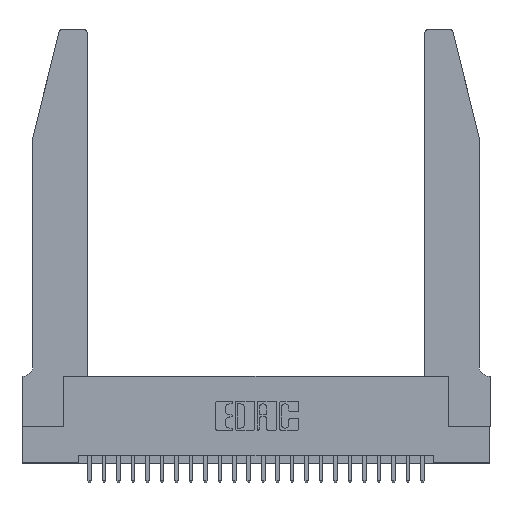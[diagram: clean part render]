
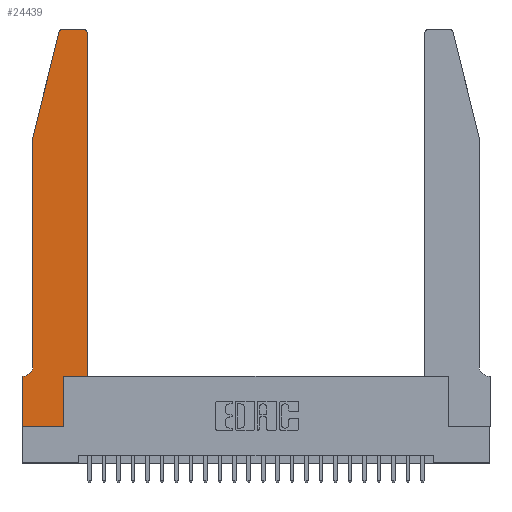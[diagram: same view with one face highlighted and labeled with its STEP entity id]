
A CAD part, top view. The second image highlights one B-rep face of the part: STEP entity #24439.
In plain terms, the highlighted planar face has unit normal (0, 0, 1).
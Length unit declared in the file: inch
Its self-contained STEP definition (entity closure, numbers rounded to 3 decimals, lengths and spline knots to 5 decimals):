
#149 = CARTESIAN_POINT ( 'NONE',  ( 0.4205, 2.75, 0.37 ) ) ;
#637 = VERTEX_POINT ( 'NONE', #7300 ) ;
#642 = AXIS2_PLACEMENT_3D ( 'NONE', #14940, #10970, #20933 ) ;
#1613 = VECTOR ( 'NONE', #25043, 39.37008 ) ;
#1618 = DIRECTION ( 'NONE',  ( 1., 0., 0. ) ) ;
#1710 = VECTOR ( 'NONE', #6680, 39.37008 ) ;
#2078 = EDGE_CURVE ( 'NONE', #21010, #8955, #11226, .T. ) ;
#2170 = CARTESIAN_POINT ( 'NONE',  ( 0., 0.35, 0.37 ) ) ;
#2839 = LINE ( 'NONE', #24958, #12929 ) ;
#3309 = DIRECTION ( 'NONE',  ( 0., 0., -1. ) ) ;
#3451 = VERTEX_POINT ( 'NONE', #17751 ) ;
#3576 = DIRECTION ( 'NONE',  ( -1., 0., 0. ) ) ;
#4223 = EDGE_CURVE ( 'NONE', #8955, #25640, #12965, .T. ) ;
#4373 = CARTESIAN_POINT ( 'NONE',  ( 0.2865, 0.35, 0.37 ) ) ;
#4541 = VECTOR ( 'NONE', #18914, 39.37008 ) ;
#4555 = AXIS2_PLACEMENT_3D ( 'NONE', #10861, #18971, #19320 ) ;
#5529 = CARTESIAN_POINT ( 'NONE',  ( 0.0755, 2., 0.37 ) ) ;
#5613 = EDGE_CURVE ( 'NONE', #10034, #25306, #20818, .T. ) ;
#5662 = CARTESIAN_POINT ( 'NONE',  ( 0.284, 2.75, 0.37 ) ) ;
#6236 = LINE ( 'NONE', #5529, #16347 ) ;
#6680 = DIRECTION ( 'NONE',  ( 0., 1., 0. ) ) ;
#6697 = VECTOR ( 'NONE', #3576, 39.37008 ) ;
#6844 = EDGE_CURVE ( 'NONE', #18125, #24211, #19316, .T. ) ;
#7100 = CARTESIAN_POINT ( 'NONE',  ( 0.2865, 0., 0.37 ) ) ;
#7226 = AXIS2_PLACEMENT_3D ( 'NONE', #2170, #18486, #14240 ) ;
#7234 = CARTESIAN_POINT ( 'NONE',  ( 0.0055, 0.42, 0.37 ) ) ;
#7300 = CARTESIAN_POINT ( 'NONE',  ( 0.0755, 2., 0.37 ) ) ;
#7358 = PLANE ( 'NONE',  #7226 ) ;
#7670 = ORIENTED_EDGE ( 'NONE', *, *, #10419, .T. ) ;
#7861 = AXIS2_PLACEMENT_3D ( 'NONE', #7234, #3309, #21483 ) ;
#7967 = LINE ( 'NONE', #15758, #6697 ) ;
#8093 = CARTESIAN_POINT ( 'NONE',  ( 0.0755, 0.35, 0.37 ) ) ;
#8360 = EDGE_CURVE ( 'NONE', #25306, #24213, #19548, .T. ) ;
#8680 = CARTESIAN_POINT ( 'NONE',  ( 0.25487, 2.72718, 0.37 ) ) ;
#8682 = ORIENTED_EDGE ( 'NONE', *, *, #2078, .T. ) ;
#8781 = ORIENTED_EDGE ( 'NONE', *, *, #20488, .T. ) ;
#8790 = ORIENTED_EDGE ( 'NONE', *, *, #19076, .T. ) ;
#8955 = VERTEX_POINT ( 'NONE', #16636 ) ;
#9292 = DIRECTION ( 'NONE',  ( 0., 1., 0. ) ) ;
#9666 = CIRCLE ( 'NONE', #4555, 0.03 ) ;
#9838 = FACE_OUTER_BOUND ( 'NONE', #14586, .T. ) ;
#10034 = VERTEX_POINT ( 'NONE', #7100 ) ;
#10419 = EDGE_CURVE ( 'NONE', #22791, #20185, #9666, .T. ) ;
#10783 = DIRECTION ( 'NONE',  ( 1., 0., 0. ) ) ;
#10861 = CARTESIAN_POINT ( 'NONE',  ( 0.4205, 2.72, 0.37 ) ) ;
#10890 = ORIENTED_EDGE ( 'NONE', *, *, #8360, .T. ) ;
#10970 = DIRECTION ( 'NONE',  ( 0., 0., 1. ) ) ;
#11226 = LINE ( 'NONE', #8093, #4541 ) ;
#11276 = DIRECTION ( 'NONE',  ( 0., -1., 0. ) ) ;
#11474 = EDGE_CURVE ( 'NONE', #3451, #21010, #26013, .T. ) ;
#12108 = EDGE_CURVE ( 'NONE', #24213, #22791, #19376, .T. ) ;
#12929 = VECTOR ( 'NONE', #11276, 39.37008 ) ;
#12965 = LINE ( 'NONE', #19267, #1613 ) ;
#13298 = DIRECTION ( 'NONE',  ( -0.239, -0.971, 0. ) ) ;
#13448 = ORIENTED_EDGE ( 'NONE', *, *, #4223, .T. ) ;
#13584 = ORIENTED_EDGE ( 'NONE', *, *, #5613, .T. ) ;
#14240 = DIRECTION ( 'NONE',  ( 1., 0., 0. ) ) ;
#14586 = EDGE_LOOP ( 'NONE', ( #8790, #24804, #21444, #8781, #20451, #8682, #13448, #21545, #13584, #10890, #24182, #7670 ) ) ;
#14940 = CARTESIAN_POINT ( 'NONE',  ( 0.284, 2.72, 0.37 ) ) ;
#15050 = CARTESIAN_POINT ( 'NONE',  ( 0.4505, 0.35, 0.37 ) ) ;
#15729 = CARTESIAN_POINT ( 'NONE',  ( 0., 0., 0.37 ) ) ;
#15758 = CARTESIAN_POINT ( 'NONE',  ( 0.2605, 2.75, 0.37 ) ) ;
#16347 = VECTOR ( 'NONE', #13298, 39.37008 ) ;
#16636 = CARTESIAN_POINT ( 'NONE',  ( 0., 0.35, 0.37 ) ) ;
#17296 = CARTESIAN_POINT ( 'NONE',  ( 0., 0., 0.37 ) ) ;
#17751 = CARTESIAN_POINT ( 'NONE',  ( 0.0755, 0.42, 0.37 ) ) ;
#18125 = VERTEX_POINT ( 'NONE', #5662 ) ;
#18486 = DIRECTION ( 'NONE',  ( 0., 0., 1. ) ) ;
#18597 = VECTOR ( 'NONE', #10783, 39.37008 ) ;
#18914 = DIRECTION ( 'NONE',  ( -1., 0., 0. ) ) ;
#18971 = DIRECTION ( 'NONE',  ( 0., 0., 1. ) ) ;
#19076 = EDGE_CURVE ( 'NONE', #20185, #18125, #7967, .T. ) ;
#19267 = CARTESIAN_POINT ( 'NONE',  ( 0., 0., 0.37 ) ) ;
#19316 = CIRCLE ( 'NONE', #642, 0.03 ) ;
#19320 = DIRECTION ( 'NONE',  ( 1., 0., 0. ) ) ;
#19331 = CARTESIAN_POINT ( 'NONE',  ( 0.2865, 0.35, 0.37 ) ) ;
#19376 = LINE ( 'NONE', #15050, #1710 ) ;
#19548 = LINE ( 'NONE', #22826, #18597 ) ;
#19781 = EDGE_CURVE ( 'NONE', #25640, #10034, #21165, .T. ) ;
#20185 = VERTEX_POINT ( 'NONE', #149 ) ;
#20211 = CARTESIAN_POINT ( 'NONE',  ( 0.0055, 0.35, 0.37 ) ) ;
#20451 = ORIENTED_EDGE ( 'NONE', *, *, #11474, .T. ) ;
#20488 = EDGE_CURVE ( 'NONE', #637, #3451, #2839, .T. ) ;
#20818 = LINE ( 'NONE', #19331, #21463 ) ;
#20933 = DIRECTION ( 'NONE',  ( 1., 0., 0. ) ) ;
#21010 = VERTEX_POINT ( 'NONE', #20211 ) ;
#21165 = LINE ( 'NONE', #15729, #22401 ) ;
#21400 = EDGE_CURVE ( 'NONE', #24211, #637, #6236, .T. ) ;
#21444 = ORIENTED_EDGE ( 'NONE', *, *, #21400, .T. ) ;
#21463 = VECTOR ( 'NONE', #9292, 39.37008 ) ;
#21483 = DIRECTION ( 'NONE',  ( -1., 0., 0. ) ) ;
#21545 = ORIENTED_EDGE ( 'NONE', *, *, #19781, .T. ) ;
#22401 = VECTOR ( 'NONE', #1618, 39.37008 ) ;
#22741 = CARTESIAN_POINT ( 'NONE',  ( 0.4505, 0.35, 0.37 ) ) ;
#22791 = VERTEX_POINT ( 'NONE', #24632 ) ;
#22826 = CARTESIAN_POINT ( 'NONE',  ( 0.4505, 0.35, 0.37 ) ) ;
#24182 = ORIENTED_EDGE ( 'NONE', *, *, #12108, .T. ) ;
#24211 = VERTEX_POINT ( 'NONE', #8680 ) ;
#24213 = VERTEX_POINT ( 'NONE', #22741 ) ;
#24439 = ADVANCED_FACE ( 'NONE', ( #9838 ), #7358, .T. ) ;
#24632 = CARTESIAN_POINT ( 'NONE',  ( 0.4505, 2.72, 0.37 ) ) ;
#24804 = ORIENTED_EDGE ( 'NONE', *, *, #6844, .T. ) ;
#24958 = CARTESIAN_POINT ( 'NONE',  ( 0.0755, 2., 0.37 ) ) ;
#25043 = DIRECTION ( 'NONE',  ( 0., -1., 0. ) ) ;
#25306 = VERTEX_POINT ( 'NONE', #4373 ) ;
#25640 = VERTEX_POINT ( 'NONE', #17296 ) ;
#26013 = CIRCLE ( 'NONE', #7861, 0.07 ) ;
